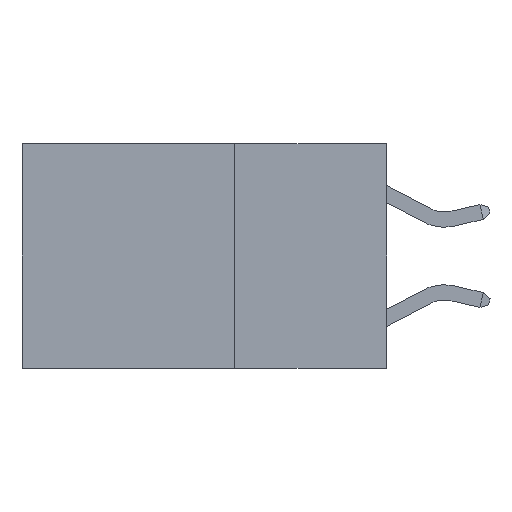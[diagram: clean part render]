
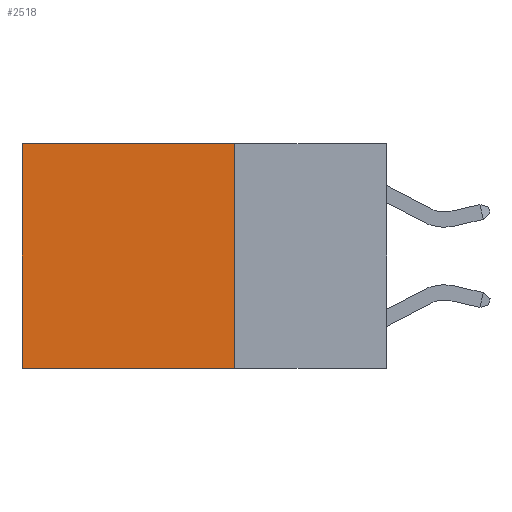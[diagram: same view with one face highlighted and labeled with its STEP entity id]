
A CAD part, left-side view. The second image highlights one B-rep face of the part: STEP entity #2518.
In plain terms, the highlighted planar face has unit normal (-1, 0, 0).
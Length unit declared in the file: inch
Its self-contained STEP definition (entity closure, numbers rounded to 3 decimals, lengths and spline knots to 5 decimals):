
#104 = CARTESIAN_POINT ( 'NONE',  ( 0.2625, 0.6, 0. ) ) ;
#131 = ORIENTED_EDGE ( 'NONE', *, *, #13121, .F. ) ;
#323 = ORIENTED_EDGE ( 'NONE', *, *, #14611, .F. ) ;
#1033 = LINE ( 'NONE', #5482, #17636 ) ;
#1107 = LINE ( 'NONE', #7125, #8714 ) ;
#2412 = DIRECTION ( 'NONE',  ( 0., 0., -1. ) ) ;
#2518 = ADVANCED_FACE ( 'NONE', ( #9936 ), #6082, .F. ) ;
#2685 = LINE ( 'NONE', #9437, #17040 ) ;
#3356 = EDGE_CURVE ( 'NONE', #14031, #17350, #1107, .T. ) ;
#4424 = DIRECTION ( 'NONE',  ( 0., 0., -1. ) ) ;
#5482 = CARTESIAN_POINT ( 'NONE',  ( 0.2625, 0.25, 0. ) ) ;
#5613 = VECTOR ( 'NONE', #8257, 39.37008 ) ;
#5997 = DIRECTION ( 'NONE',  ( 1., 0., 0. ) ) ;
#6082 = PLANE ( 'NONE',  #13772 ) ;
#6769 = EDGE_LOOP ( 'NONE', ( #7582, #323, #131, #8059 ) ) ;
#6952 = CARTESIAN_POINT ( 'NONE',  ( 0.2625, 0.25, -0.37 ) ) ;
#7125 = CARTESIAN_POINT ( 'NONE',  ( 0.2625, 0.25, 0. ) ) ;
#7553 = VERTEX_POINT ( 'NONE', #9369 ) ;
#7582 = ORIENTED_EDGE ( 'NONE', *, *, #11122, .T. ) ;
#7910 = CARTESIAN_POINT ( 'NONE',  ( 0.2625, 0.25, 0. ) ) ;
#8059 = ORIENTED_EDGE ( 'NONE', *, *, #3356, .T. ) ;
#8257 = DIRECTION ( 'NONE',  ( 0., 1., 0. ) ) ;
#8506 = DIRECTION ( 'NONE',  ( 0., 1., 0. ) ) ;
#8714 = VECTOR ( 'NONE', #8506, 39.37008 ) ;
#9369 = CARTESIAN_POINT ( 'NONE',  ( 0.2625, 0.6, -0.37 ) ) ;
#9437 = CARTESIAN_POINT ( 'NONE',  ( 0.2625, 0.6, 0. ) ) ;
#9608 = LINE ( 'NONE', #6952, #5613 ) ;
#9936 = FACE_OUTER_BOUND ( 'NONE', #6769, .T. ) ;
#11122 = EDGE_CURVE ( 'NONE', #17350, #7553, #2685, .T. ) ;
#12664 = DIRECTION ( 'NONE',  ( 0., 0., -1. ) ) ;
#12987 = CARTESIAN_POINT ( 'NONE',  ( 0.2625, 0.25, 0. ) ) ;
#13121 = EDGE_CURVE ( 'NONE', #14031, #14935, #1033, .T. ) ;
#13632 = CARTESIAN_POINT ( 'NONE',  ( 0.2625, 0.25, -0.37 ) ) ;
#13772 = AXIS2_PLACEMENT_3D ( 'NONE', #12987, #5997, #4424 ) ;
#14031 = VERTEX_POINT ( 'NONE', #7910 ) ;
#14611 = EDGE_CURVE ( 'NONE', #14935, #7553, #9608, .T. ) ;
#14935 = VERTEX_POINT ( 'NONE', #13632 ) ;
#17040 = VECTOR ( 'NONE', #2412, 39.37008 ) ;
#17350 = VERTEX_POINT ( 'NONE', #104 ) ;
#17636 = VECTOR ( 'NONE', #12664, 39.37008 ) ;
